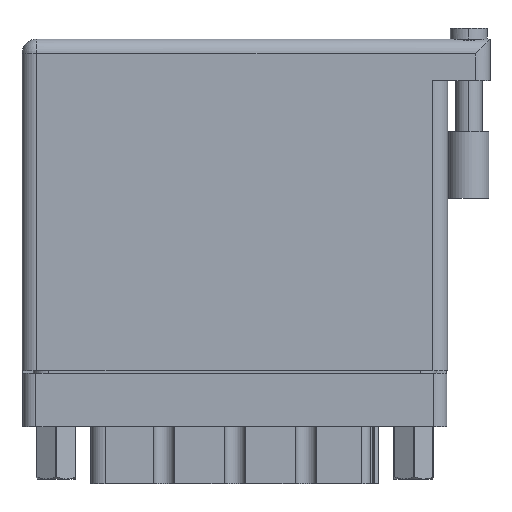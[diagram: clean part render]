
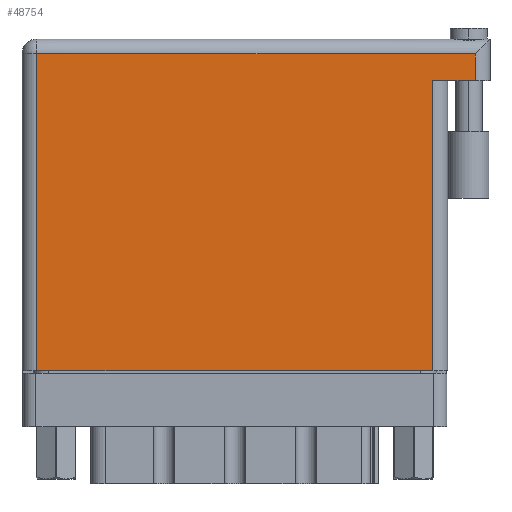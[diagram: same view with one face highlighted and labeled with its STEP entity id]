
A CAD part, front view. The second image highlights one B-rep face of the part: STEP entity #48754.
In plain terms, the highlighted face is planar.
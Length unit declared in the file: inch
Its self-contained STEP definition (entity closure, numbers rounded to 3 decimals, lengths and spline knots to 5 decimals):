
#977 = ORIENTED_EDGE ( 'NONE', *, *, #30873, .T. ) ;
#2300 = VECTOR ( 'NONE', #28000, 39.37008 ) ;
#2537 = DIRECTION ( 'NONE',  ( 0., -1., 0. ) ) ;
#2718 = CARTESIAN_POINT ( 'NONE',  ( 0., 1.566, 0. ) ) ;
#5068 = CARTESIAN_POINT ( 'NONE',  ( 1.938, 1.369, 0. ) ) ;
#5740 = VECTOR ( 'NONE', #5908, 39.37008 ) ;
#5908 = DIRECTION ( 'NONE',  ( 0., 1., 0. ) ) ;
#8532 = FACE_OUTER_BOUND ( 'NONE', #40932, .T. ) ;
#10897 = EDGE_CURVE ( 'NONE', #42690, #18132, #48006, .T. ) ;
#11209 = VECTOR ( 'NONE', #24943, 39.37008 ) ;
#11688 = DIRECTION ( 'NONE',  ( -1., 0., 0. ) ) ;
#12141 = CARTESIAN_POINT ( 'NONE',  ( 0., 0., 0. ) ) ;
#12342 = VECTOR ( 'NONE', #17307, 39.37008 ) ;
#13495 = VERTEX_POINT ( 'NONE', #45792 ) ;
#13731 = CARTESIAN_POINT ( 'NONE',  ( 1.938, 1.369, 0. ) ) ;
#16746 = ORIENTED_EDGE ( 'NONE', *, *, #32294, .F. ) ;
#17223 = DIRECTION ( 'NONE',  ( 0., 0., -1. ) ) ;
#17307 = DIRECTION ( 'NONE',  ( 0., 1., 0. ) ) ;
#17996 = VECTOR ( 'NONE', #11688, 39.37008 ) ;
#18132 = VERTEX_POINT ( 'NONE', #43823 ) ;
#24659 = VERTEX_POINT ( 'NONE', #42648 ) ;
#24943 = DIRECTION ( 'NONE',  ( -1., 0., 0. ) ) ;
#26515 = AXIS2_PLACEMENT_3D ( 'NONE', #2718, #17223, #40371 ) ;
#26802 = LINE ( 'NONE', #12141, #2300 ) ;
#28000 = DIRECTION ( 'NONE',  ( 1., 0., 0. ) ) ;
#30873 = EDGE_CURVE ( 'NONE', #18132, #24659, #36408, .T. ) ;
#31379 = EDGE_CURVE ( 'NONE', #24659, #47849, #26802, .T. ) ;
#31826 = ORIENTED_EDGE ( 'NONE', *, *, #32838, .T. ) ;
#32294 = EDGE_CURVE ( 'NONE', #13495, #34600, #41100, .T. ) ;
#32838 = EDGE_CURVE ( 'NONE', #13495, #42690, #43482, .T. ) ;
#34600 = VERTEX_POINT ( 'NONE', #5068 ) ;
#36278 = LINE ( 'NONE', #13731, #5740 ) ;
#36374 = CARTESIAN_POINT ( 'NONE',  ( 2.208, 1.369, 0. ) ) ;
#36408 = LINE ( 'NONE', #47899, #46060 ) ;
#38025 = CARTESIAN_POINT ( 'NONE',  ( 2.138, 1.496, 0. ) ) ;
#40371 = DIRECTION ( 'NONE',  ( -1., 0., 0. ) ) ;
#40932 = EDGE_LOOP ( 'NONE', ( #47585, #41181, #16746, #31826, #48798, #977 ) ) ;
#40995 = CARTESIAN_POINT ( 'NONE',  ( 1.938, 0., 0. ) ) ;
#41100 = LINE ( 'NONE', #36374, #11209 ) ;
#41181 = ORIENTED_EDGE ( 'NONE', *, *, #43087, .T. ) ;
#42648 = CARTESIAN_POINT ( 'NONE',  ( 0.07, 0., 0. ) ) ;
#42690 = VERTEX_POINT ( 'NONE', #38025 ) ;
#42996 = CARTESIAN_POINT ( 'NONE',  ( 0., 1.496, 0. ) ) ;
#43087 = EDGE_CURVE ( 'NONE', #47849, #34600, #36278, .T. ) ;
#43482 = LINE ( 'NONE', #43490, #12342 ) ;
#43490 = CARTESIAN_POINT ( 'NONE',  ( 2.138, 1.566, 0. ) ) ;
#43823 = CARTESIAN_POINT ( 'NONE',  ( 0.07, 1.496, 0. ) ) ;
#45792 = CARTESIAN_POINT ( 'NONE',  ( 2.138, 1.369, 0. ) ) ;
#46060 = VECTOR ( 'NONE', #2537, 39.37008 ) ;
#47585 = ORIENTED_EDGE ( 'NONE', *, *, #31379, .T. ) ;
#47849 = VERTEX_POINT ( 'NONE', #40995 ) ;
#47899 = CARTESIAN_POINT ( 'NONE',  ( 0.07, 0., 0. ) ) ;
#48006 = LINE ( 'NONE', #42996, #17996 ) ;
#48076 = PLANE ( 'NONE',  #26515 ) ;
#48754 = ADVANCED_FACE ( 'NONE', ( #8532 ), #48076, .F. ) ;
#48798 = ORIENTED_EDGE ( 'NONE', *, *, #10897, .T. ) ;
